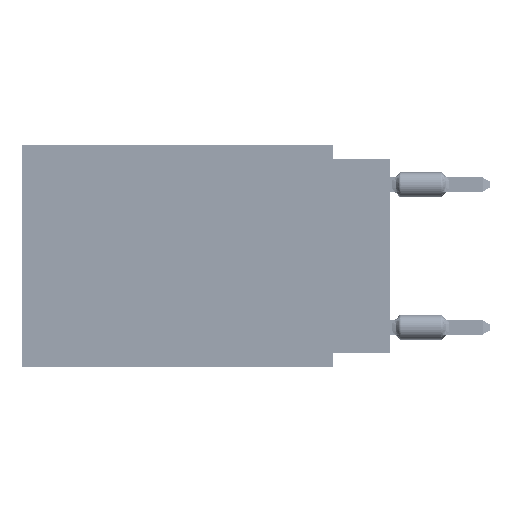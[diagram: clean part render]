
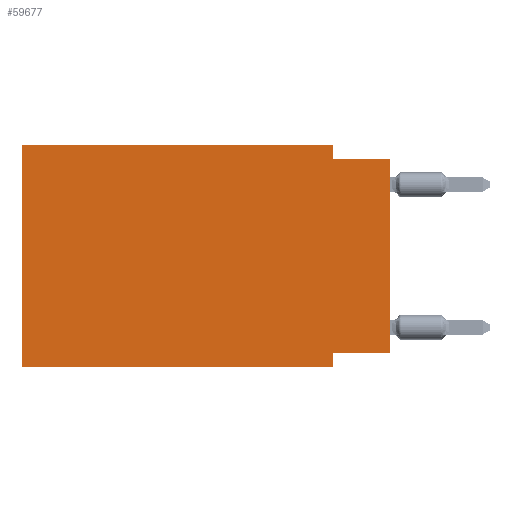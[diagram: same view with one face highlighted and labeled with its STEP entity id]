
A CAD part, left-side view. The second image highlights one B-rep face of the part: STEP entity #59677.
In plain terms, the highlighted planar face has unit normal (-1, 0, 0).
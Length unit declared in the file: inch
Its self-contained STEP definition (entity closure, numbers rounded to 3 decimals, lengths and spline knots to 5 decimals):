
#4626 = EDGE_CURVE ( 'NONE', #60147, #28745, #42059, .T. ) ;
#5000 = DIRECTION ( 'NONE',  ( 0., -1., 0. ) ) ;
#5472 = LINE ( 'NONE', #25358, #20877 ) ;
#5703 = VERTEX_POINT ( 'NONE', #45833 ) ;
#6104 = CARTESIAN_POINT ( 'NONE',  ( 0., 0.1, -0.39 ) ) ;
#6746 = VECTOR ( 'NONE', #22686, 39.37008 ) ;
#6930 = CARTESIAN_POINT ( 'NONE',  ( 0., 0., -0.365 ) ) ;
#7488 = VERTEX_POINT ( 'NONE', #53664 ) ;
#8441 = CARTESIAN_POINT ( 'NONE',  ( 0., 0.645, -0.39 ) ) ;
#11915 = VECTOR ( 'NONE', #32788, 39.37008 ) ;
#11925 = DIRECTION ( 'NONE',  ( 0., 0., 1. ) ) ;
#12064 = LINE ( 'NONE', #6930, #6746 ) ;
#14863 = VERTEX_POINT ( 'NONE', #51946 ) ;
#15305 = AXIS2_PLACEMENT_3D ( 'NONE', #52499, #16426, #37042 ) ;
#15704 = EDGE_LOOP ( 'NONE', ( #56883, #50824, #46259, #27268, #31313, #28302, #41201, #55442 ) ) ;
#16426 = DIRECTION ( 'NONE',  ( 1., 0., 0. ) ) ;
#16527 = EDGE_CURVE ( 'NONE', #44259, #5703, #26359, .T. ) ;
#16623 = EDGE_CURVE ( 'NONE', #16788, #5703, #50001, .T. ) ;
#16788 = VERTEX_POINT ( 'NONE', #8441 ) ;
#18257 = CARTESIAN_POINT ( 'NONE',  ( 0., 0.1, -0.365 ) ) ;
#20877 = VECTOR ( 'NONE', #26391, 39.37008 ) ;
#21232 = EDGE_CURVE ( 'NONE', #14863, #44259, #12064, .T. ) ;
#22686 = DIRECTION ( 'NONE',  ( 0., 1., 0. ) ) ;
#24803 = VERTEX_POINT ( 'NONE', #25303 ) ;
#25303 = CARTESIAN_POINT ( 'NONE',  ( 0., 0.645, 0. ) ) ;
#25358 = CARTESIAN_POINT ( 'NONE',  ( 0., 0.645, 0. ) ) ;
#26359 = LINE ( 'NONE', #6104, #51406 ) ;
#26391 = DIRECTION ( 'NONE',  ( 0., -1., 0. ) ) ;
#27268 = ORIENTED_EDGE ( 'NONE', *, *, #51389, .F. ) ;
#28302 = ORIENTED_EDGE ( 'NONE', *, *, #16623, .T. ) ;
#28745 = VERTEX_POINT ( 'NONE', #35843 ) ;
#31313 = ORIENTED_EDGE ( 'NONE', *, *, #47984, .F. ) ;
#31542 = PLANE ( 'NONE',  #15305 ) ;
#32788 = DIRECTION ( 'NONE',  ( 0., 0., 1. ) ) ;
#33210 = LINE ( 'NONE', #39378, #54533 ) ;
#34981 = VECTOR ( 'NONE', #49672, 39.37008 ) ;
#35843 = CARTESIAN_POINT ( 'NONE',  ( 0., 0., -0.025 ) ) ;
#37042 = DIRECTION ( 'NONE',  ( 0., 0., -1. ) ) ;
#37076 = VECTOR ( 'NONE', #5000, 39.37008 ) ;
#37960 = CARTESIAN_POINT ( 'NONE',  ( 0., 0.1, -0.025 ) ) ;
#39216 = VECTOR ( 'NONE', #61337, 39.37008 ) ;
#39378 = CARTESIAN_POINT ( 'NONE',  ( 0., 0., 0. ) ) ;
#41201 = ORIENTED_EDGE ( 'NONE', *, *, #16527, .F. ) ;
#42059 = LINE ( 'NONE', #52029, #37076 ) ;
#42773 = LINE ( 'NONE', #47588, #11915 ) ;
#44259 = VERTEX_POINT ( 'NONE', #18257 ) ;
#44847 = CARTESIAN_POINT ( 'NONE',  ( 0., 0.645, -0.39 ) ) ;
#45833 = CARTESIAN_POINT ( 'NONE',  ( 0., 0.1, -0.39 ) ) ;
#46259 = ORIENTED_EDGE ( 'NONE', *, *, #46506, .F. ) ;
#46506 = EDGE_CURVE ( 'NONE', #7488, #60147, #65484, .T. ) ;
#47588 = CARTESIAN_POINT ( 'NONE',  ( 0., 0.645, 0. ) ) ;
#47967 = DIRECTION ( 'NONE',  ( 0., 0., -1. ) ) ;
#47984 = EDGE_CURVE ( 'NONE', #16788, #24803, #42773, .T. ) ;
#49672 = DIRECTION ( 'NONE',  ( 0., -1., 0. ) ) ;
#50001 = LINE ( 'NONE', #44847, #34981 ) ;
#50824 = ORIENTED_EDGE ( 'NONE', *, *, #4626, .F. ) ;
#51389 = EDGE_CURVE ( 'NONE', #24803, #7488, #5472, .T. ) ;
#51406 = VECTOR ( 'NONE', #47967, 39.37008 ) ;
#51946 = CARTESIAN_POINT ( 'NONE',  ( 0., 0., -0.365 ) ) ;
#52029 = CARTESIAN_POINT ( 'NONE',  ( 0., 0., -0.025 ) ) ;
#52499 = CARTESIAN_POINT ( 'NONE',  ( 0., 0.645, 0. ) ) ;
#53664 = CARTESIAN_POINT ( 'NONE',  ( 0., 0.1, 0. ) ) ;
#54533 = VECTOR ( 'NONE', #11925, 39.37008 ) ;
#55442 = ORIENTED_EDGE ( 'NONE', *, *, #21232, .F. ) ;
#56883 = ORIENTED_EDGE ( 'NONE', *, *, #57239, .T. ) ;
#57239 = EDGE_CURVE ( 'NONE', #14863, #28745, #33210, .T. ) ;
#57984 = FACE_OUTER_BOUND ( 'NONE', #15704, .T. ) ;
#59677 = ADVANCED_FACE ( 'NONE', ( #57984 ), #31542, .F. ) ;
#60147 = VERTEX_POINT ( 'NONE', #37960 ) ;
#61337 = DIRECTION ( 'NONE',  ( 0., 0., -1. ) ) ;
#65484 = LINE ( 'NONE', #66482, #39216 ) ;
#66482 = CARTESIAN_POINT ( 'NONE',  ( 0., 0.1, 0. ) ) ;
